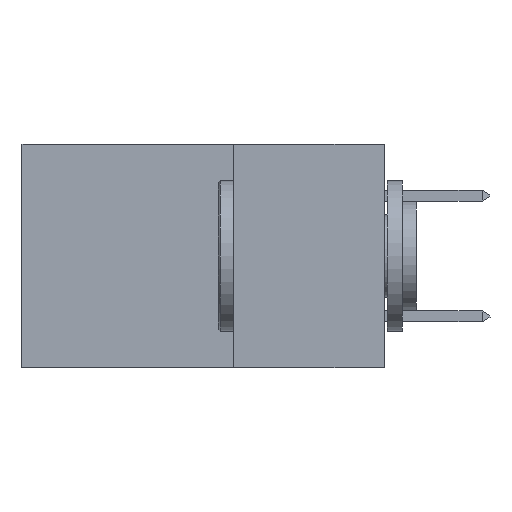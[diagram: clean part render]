
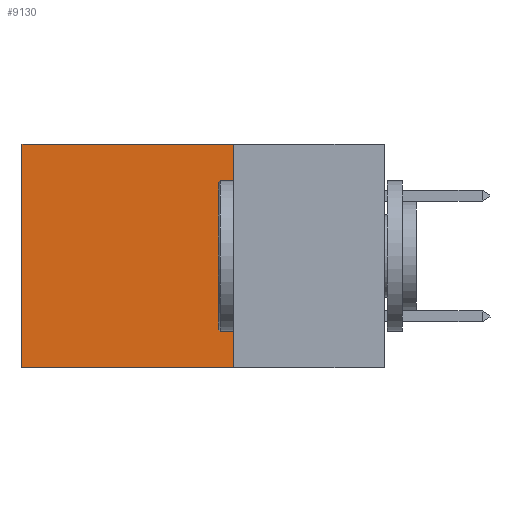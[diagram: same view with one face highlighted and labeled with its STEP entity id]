
A CAD part, left-side view. The second image highlights one B-rep face of the part: STEP entity #9130.
In plain terms, the highlighted planar face has unit normal (-1, 0, 0).
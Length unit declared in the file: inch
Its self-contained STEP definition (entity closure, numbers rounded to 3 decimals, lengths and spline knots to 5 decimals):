
#326 = CARTESIAN_POINT ( 'NONE',  ( 0.2875, 0.6, -0.37 ) ) ;
#827 = EDGE_CURVE ( 'NONE', #18180, #12901, #20775, .T. ) ;
#1186 = EDGE_CURVE ( 'NONE', #22389, #7400, #9310, .T. ) ;
#1655 = VECTOR ( 'NONE', #13418, 39.37008 ) ;
#3778 = PLANE ( 'NONE',  #6611 ) ;
#4474 = ORIENTED_EDGE ( 'NONE', *, *, #1186, .T. ) ;
#5502 = EDGE_LOOP ( 'NONE', ( #4474, #14920, #6843, #12262 ) ) ;
#5592 = DIRECTION ( 'NONE',  ( 0., 0., -1. ) ) ;
#6315 = DIRECTION ( 'NONE',  ( 0., 1., 0. ) ) ;
#6611 = AXIS2_PLACEMENT_3D ( 'NONE', #21627, #16313, #5592 ) ;
#6843 = ORIENTED_EDGE ( 'NONE', *, *, #827, .F. ) ;
#6970 = EDGE_CURVE ( 'NONE', #18180, #22389, #20430, .T. ) ;
#7400 = VERTEX_POINT ( 'NONE', #326 ) ;
#9130 = ADVANCED_FACE ( 'NONE', ( #20082 ), #3778, .F. ) ;
#9310 = LINE ( 'NONE', #18172, #10435 ) ;
#10435 = VECTOR ( 'NONE', #18244, 39.37008 ) ;
#11366 = CARTESIAN_POINT ( 'NONE',  ( 0.2875, 0.25, -0.37 ) ) ;
#12262 = ORIENTED_EDGE ( 'NONE', *, *, #6970, .T. ) ;
#12437 = DIRECTION ( 'NONE',  ( 0., 1., 0. ) ) ;
#12901 = VERTEX_POINT ( 'NONE', #11366 ) ;
#13133 = VECTOR ( 'NONE', #12437, 39.37008 ) ;
#13418 = DIRECTION ( 'NONE',  ( 0., 0., -1. ) ) ;
#13883 = EDGE_CURVE ( 'NONE', #12901, #7400, #22618, .T. ) ;
#14513 = VECTOR ( 'NONE', #6315, 39.37008 ) ;
#14920 = ORIENTED_EDGE ( 'NONE', *, *, #13883, .F. ) ;
#15178 = CARTESIAN_POINT ( 'NONE',  ( 0.2875, 0.25, 0. ) ) ;
#15933 = CARTESIAN_POINT ( 'NONE',  ( 0.2875, 0.25, -0.37 ) ) ;
#16313 = DIRECTION ( 'NONE',  ( 1., 0., 0. ) ) ;
#17750 = CARTESIAN_POINT ( 'NONE',  ( 0.2875, 0.6, 0. ) ) ;
#18172 = CARTESIAN_POINT ( 'NONE',  ( 0.2875, 0.6, 0. ) ) ;
#18180 = VERTEX_POINT ( 'NONE', #20789 ) ;
#18244 = DIRECTION ( 'NONE',  ( 0., 0., -1. ) ) ;
#20082 = FACE_OUTER_BOUND ( 'NONE', #5502, .T. ) ;
#20430 = LINE ( 'NONE', #15178, #14513 ) ;
#20775 = LINE ( 'NONE', #21263, #1655 ) ;
#20789 = CARTESIAN_POINT ( 'NONE',  ( 0.2875, 0.25, 0. ) ) ;
#21263 = CARTESIAN_POINT ( 'NONE',  ( 0.2875, 0.25, 0. ) ) ;
#21627 = CARTESIAN_POINT ( 'NONE',  ( 0.2875, 0.25, 0. ) ) ;
#22389 = VERTEX_POINT ( 'NONE', #17750 ) ;
#22618 = LINE ( 'NONE', #15933, #13133 ) ;
